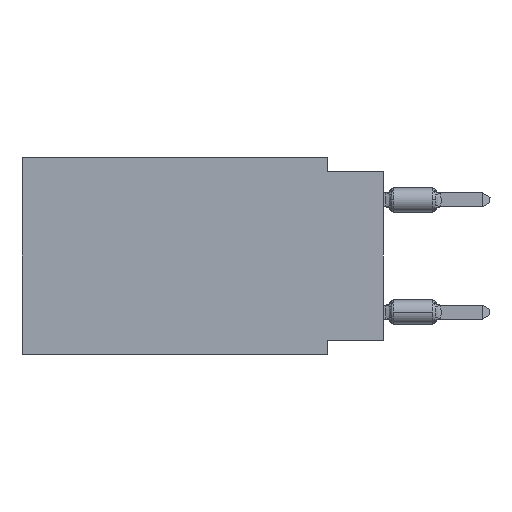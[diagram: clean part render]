
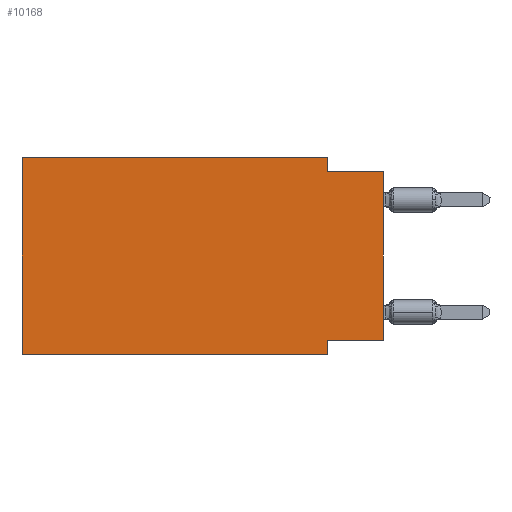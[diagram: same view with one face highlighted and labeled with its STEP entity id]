
A CAD part, left-side view. The second image highlights one B-rep face of the part: STEP entity #10168.
In plain terms, the highlighted planar face has unit normal (-1, 0, 0).
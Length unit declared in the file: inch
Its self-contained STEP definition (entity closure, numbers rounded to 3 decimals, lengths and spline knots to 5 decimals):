
#1884 = ORIENTED_EDGE ( 'NONE', *, *, #36808, .F. ) ;
#2828 = VECTOR ( 'NONE', #9204, 39.37008 ) ;
#3594 = ORIENTED_EDGE ( 'NONE', *, *, #39346, .T. ) ;
#4501 = VERTEX_POINT ( 'NONE', #9298 ) ;
#5353 = CARTESIAN_POINT ( 'NONE',  ( 0., 0.645, 0. ) ) ;
#6510 = EDGE_CURVE ( 'NONE', #23114, #4501, #44844, .T. ) ;
#7090 = LINE ( 'NONE', #39073, #34436 ) ;
#7271 = CARTESIAN_POINT ( 'NONE',  ( 0., 0., -0.325 ) ) ;
#8558 = EDGE_CURVE ( 'NONE', #41605, #12405, #34940, .T. ) ;
#9204 = DIRECTION ( 'NONE',  ( 0., 0., -1. ) ) ;
#9298 = CARTESIAN_POINT ( 'NONE',  ( 0., 0.1, -0.325 ) ) ;
#9385 = DIRECTION ( 'NONE',  ( 0., 0., -1. ) ) ;
#10168 = ADVANCED_FACE ( 'NONE', ( #17712 ), #13671, .F. ) ;
#11764 = VERTEX_POINT ( 'NONE', #19473 ) ;
#11944 = ORIENTED_EDGE ( 'NONE', *, *, #49064, .F. ) ;
#12104 = ORIENTED_EDGE ( 'NONE', *, *, #8558, .F. ) ;
#12405 = VERTEX_POINT ( 'NONE', #22447 ) ;
#12851 = CARTESIAN_POINT ( 'NONE',  ( 0., 0., -0.025 ) ) ;
#13671 = PLANE ( 'NONE',  #31433 ) ;
#14634 = CARTESIAN_POINT ( 'NONE',  ( 0., 0., -0.325 ) ) ;
#14853 = ORIENTED_EDGE ( 'NONE', *, *, #6510, .F. ) ;
#15868 = CARTESIAN_POINT ( 'NONE',  ( 0., 0.645, 0. ) ) ;
#16879 = LINE ( 'NONE', #12851, #36922 ) ;
#17712 = FACE_OUTER_BOUND ( 'NONE', #40204, .T. ) ;
#18424 = CARTESIAN_POINT ( 'NONE',  ( 0., 0.645, -0.35 ) ) ;
#19083 = CARTESIAN_POINT ( 'NONE',  ( 0., 0.645, -0.35 ) ) ;
#19202 = DIRECTION ( 'NONE',  ( 0., -1., 0. ) ) ;
#19473 = CARTESIAN_POINT ( 'NONE',  ( 0., 0.1, -0.35 ) ) ;
#21646 = EDGE_CURVE ( 'NONE', #40429, #11764, #30767, .T. ) ;
#22447 = CARTESIAN_POINT ( 'NONE',  ( 0., 0.1, -0.025 ) ) ;
#23114 = VERTEX_POINT ( 'NONE', #14634 ) ;
#24379 = DIRECTION ( 'NONE',  ( 0., 0., 1. ) ) ;
#27676 = DIRECTION ( 'NONE',  ( 0., 1., 0. ) ) ;
#27725 = VERTEX_POINT ( 'NONE', #28349 ) ;
#28226 = ORIENTED_EDGE ( 'NONE', *, *, #28806, .F. ) ;
#28349 = CARTESIAN_POINT ( 'NONE',  ( 0., 0., -0.025 ) ) ;
#28806 = EDGE_CURVE ( 'NONE', #45976, #41605, #52688, .T. ) ;
#30615 = VECTOR ( 'NONE', #32247, 39.37008 ) ;
#30767 = LINE ( 'NONE', #18424, #41639 ) ;
#31433 = AXIS2_PLACEMENT_3D ( 'NONE', #5353, #33813, #9385 ) ;
#32247 = DIRECTION ( 'NONE',  ( 0., -1., 0. ) ) ;
#32429 = LINE ( 'NONE', #49374, #49896 ) ;
#33813 = DIRECTION ( 'NONE',  ( 1., 0., 0. ) ) ;
#34389 = CARTESIAN_POINT ( 'NONE',  ( 0., 0.1, 0. ) ) ;
#34436 = VECTOR ( 'NONE', #48185, 39.37008 ) ;
#34744 = EDGE_CURVE ( 'NONE', #12405, #27725, #16879, .T. ) ;
#34940 = LINE ( 'NONE', #34389, #41579 ) ;
#36808 = EDGE_CURVE ( 'NONE', #4501, #11764, #37658, .T. ) ;
#36922 = VECTOR ( 'NONE', #45586, 39.37008 ) ;
#37647 = CARTESIAN_POINT ( 'NONE',  ( 0., 0.1, 0. ) ) ;
#37658 = LINE ( 'NONE', #41940, #2828 ) ;
#39073 = CARTESIAN_POINT ( 'NONE',  ( 0., 0.645, 0. ) ) ;
#39346 = EDGE_CURVE ( 'NONE', #23114, #27725, #32429, .T. ) ;
#40204 = EDGE_LOOP ( 'NONE', ( #3594, #41542, #12104, #28226, #11944, #48176, #1884, #14853 ) ) ;
#40429 = VERTEX_POINT ( 'NONE', #19083 ) ;
#41542 = ORIENTED_EDGE ( 'NONE', *, *, #34744, .F. ) ;
#41579 = VECTOR ( 'NONE', #50797, 39.37008 ) ;
#41605 = VERTEX_POINT ( 'NONE', #37647 ) ;
#41639 = VECTOR ( 'NONE', #19202, 39.37008 ) ;
#41940 = CARTESIAN_POINT ( 'NONE',  ( 0., 0.1, -0.35 ) ) ;
#44844 = LINE ( 'NONE', #7271, #52745 ) ;
#45586 = DIRECTION ( 'NONE',  ( 0., -1., 0. ) ) ;
#45976 = VERTEX_POINT ( 'NONE', #47897 ) ;
#47897 = CARTESIAN_POINT ( 'NONE',  ( 0., 0.645, 0. ) ) ;
#48176 = ORIENTED_EDGE ( 'NONE', *, *, #21646, .T. ) ;
#48185 = DIRECTION ( 'NONE',  ( 0., 0., 1. ) ) ;
#49064 = EDGE_CURVE ( 'NONE', #40429, #45976, #7090, .T. ) ;
#49374 = CARTESIAN_POINT ( 'NONE',  ( 0., 0., 0. ) ) ;
#49896 = VECTOR ( 'NONE', #24379, 39.37008 ) ;
#50797 = DIRECTION ( 'NONE',  ( 0., 0., -1. ) ) ;
#52688 = LINE ( 'NONE', #15868, #30615 ) ;
#52745 = VECTOR ( 'NONE', #27676, 39.37008 ) ;
